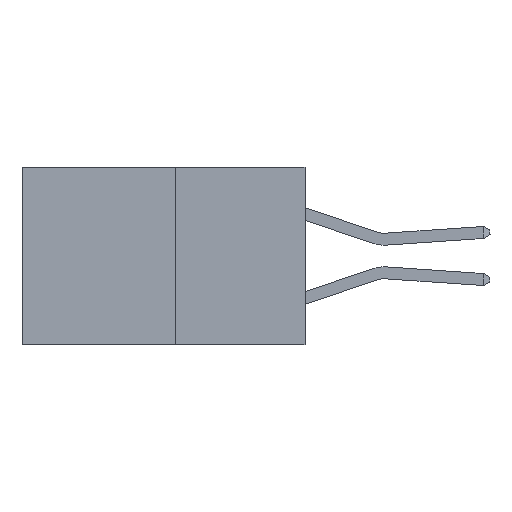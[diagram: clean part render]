
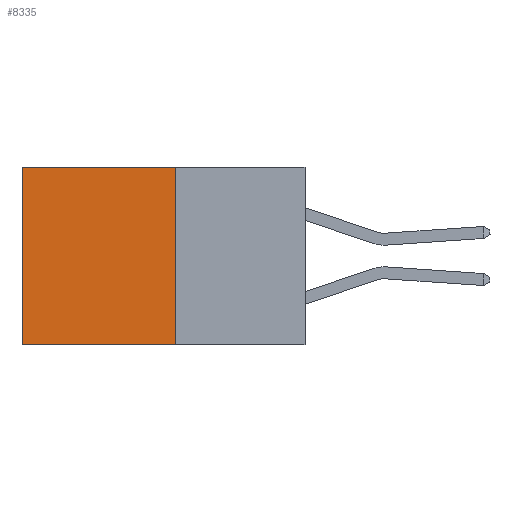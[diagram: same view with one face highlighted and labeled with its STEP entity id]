
A CAD part, left-side view. The second image highlights one B-rep face of the part: STEP entity #8335.
In plain terms, the highlighted planar face has unit normal (-1, 0, 0).
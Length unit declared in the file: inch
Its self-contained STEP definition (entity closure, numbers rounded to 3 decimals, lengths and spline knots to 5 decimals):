
#10 = ORIENTED_EDGE ( 'NONE', *, *, #11633, .T. ) ;
#116 = EDGE_CURVE ( 'NONE', #5427, #14615, #2739, .T. ) ;
#226 = ORIENTED_EDGE ( 'NONE', *, *, #14581, .F. ) ;
#1152 = ORIENTED_EDGE ( 'NONE', *, *, #9019, .F. ) ;
#1568 = CARTESIAN_POINT ( 'NONE',  ( 0.277, 0.59, 0. ) ) ;
#1885 = CARTESIAN_POINT ( 'NONE',  ( 0.277, 0.27, -0.37 ) ) ;
#1967 = VECTOR ( 'NONE', #12846, 39.37008 ) ;
#2160 = ORIENTED_EDGE ( 'NONE', *, *, #116, .T. ) ;
#2176 = FACE_OUTER_BOUND ( 'NONE', #7039, .T. ) ;
#2739 = LINE ( 'NONE', #3009, #12131 ) ;
#3009 = CARTESIAN_POINT ( 'NONE',  ( 0.277, 0.27, 0. ) ) ;
#3870 = DIRECTION ( 'NONE',  ( 0., 1., 0. ) ) ;
#4369 = DIRECTION ( 'NONE',  ( 0., 0., -1. ) ) ;
#5427 = VERTEX_POINT ( 'NONE', #11706 ) ;
#6800 = LINE ( 'NONE', #13698, #12867 ) ;
#7039 = EDGE_LOOP ( 'NONE', ( #10, #226, #1152, #2160 ) ) ;
#7041 = DIRECTION ( 'NONE',  ( 0., 0., -1. ) ) ;
#7670 = DIRECTION ( 'NONE',  ( 0., 1., 0. ) ) ;
#7760 = VERTEX_POINT ( 'NONE', #11191 ) ;
#8030 = PLANE ( 'NONE',  #14200 ) ;
#8335 = ADVANCED_FACE ( 'NONE', ( #2176 ), #8030, .F. ) ;
#8518 = LINE ( 'NONE', #14018, #1967 ) ;
#9019 = EDGE_CURVE ( 'NONE', #5427, #10586, #8518, .T. ) ;
#9176 = LINE ( 'NONE', #14254, #12407 ) ;
#10586 = VERTEX_POINT ( 'NONE', #10866 ) ;
#10866 = CARTESIAN_POINT ( 'NONE',  ( 0.277, 0.27, -0.37 ) ) ;
#11191 = CARTESIAN_POINT ( 'NONE',  ( 0.277, 0.59, -0.37 ) ) ;
#11633 = EDGE_CURVE ( 'NONE', #14615, #7760, #9176, .T. ) ;
#11669 = DIRECTION ( 'NONE',  ( 1., 0., 0. ) ) ;
#11706 = CARTESIAN_POINT ( 'NONE',  ( 0.277, 0.27, 0. ) ) ;
#12131 = VECTOR ( 'NONE', #3870, 39.37008 ) ;
#12407 = VECTOR ( 'NONE', #7041, 39.37008 ) ;
#12846 = DIRECTION ( 'NONE',  ( 0., 0., -1. ) ) ;
#12867 = VECTOR ( 'NONE', #7670, 39.37008 ) ;
#13698 = CARTESIAN_POINT ( 'NONE',  ( 0.277, 0.27, -0.37 ) ) ;
#14018 = CARTESIAN_POINT ( 'NONE',  ( 0.277, 0.27, -0.37 ) ) ;
#14200 = AXIS2_PLACEMENT_3D ( 'NONE', #1885, #11669, #4369 ) ;
#14254 = CARTESIAN_POINT ( 'NONE',  ( 0.277, 0.59, -0.37 ) ) ;
#14581 = EDGE_CURVE ( 'NONE', #10586, #7760, #6800, .T. ) ;
#14615 = VERTEX_POINT ( 'NONE', #1568 ) ;
